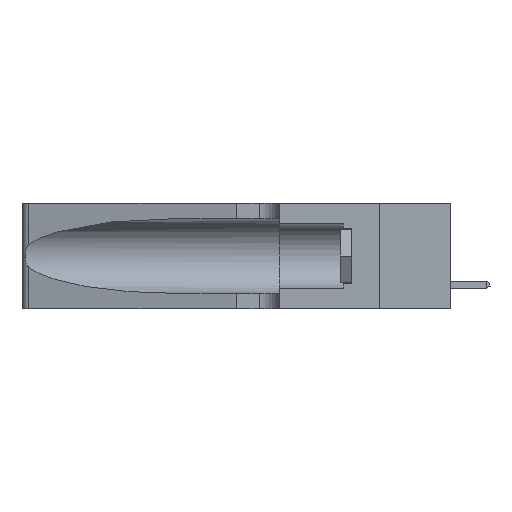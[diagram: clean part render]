
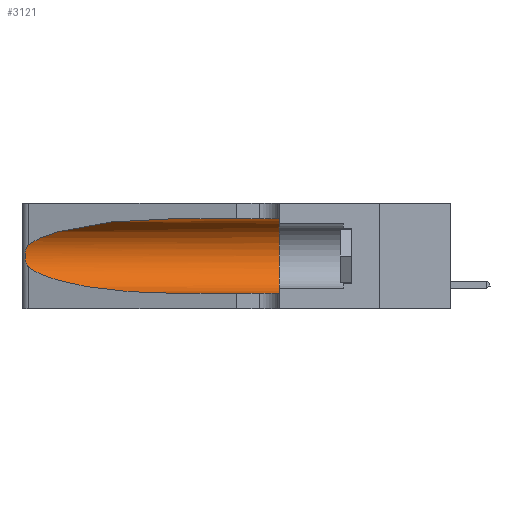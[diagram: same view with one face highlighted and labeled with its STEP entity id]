
A CAD part, left-side view. The second image highlights one B-rep face of the part: STEP entity #3121.
In plain terms, the highlighted cylindrical face has radius 3.308 mm (diameter 6.617 mm), a partial arc.
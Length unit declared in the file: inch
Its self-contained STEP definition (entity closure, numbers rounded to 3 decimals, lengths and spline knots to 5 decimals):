
#1227 = DIRECTION ( 'NONE',  ( 0., 1., 0. ) ) ;
#1298 = CYLINDRICAL_SURFACE ( 'NONE', #15451, 0.13025 ) ;
#1699 = CARTESIAN_POINT ( 'NONE',  ( 0.1305, 0.35, 0.05475 ) ) ;
#2047 = VERTEX_POINT ( 'NONE', #17541 ) ;
#2241 = ORIENTED_EDGE ( 'NONE', *, *, #7390, .F. ) ;
#3095 = CARTESIAN_POINT ( 'NONE',  ( 0.25487, 1.22718, 0.14631 ) ) ;
#3121 = ADVANCED_FACE ( 'NONE', ( #20986 ), #1298, .F. ) ;
#3146 = CARTESIAN_POINT ( 'NONE',  ( 0.18966, 0.96281, 0.05475 ) ) ;
#3394 = CARTESIAN_POINT ( 'NONE',  ( 0.25487, 1.22718, 0.22369 ) ) ;
#3983 = LINE ( 'NONE', #20571, #10694 ) ;
#4191 = CARTESIAN_POINT ( 'NONE',  ( 0.1305, 0.35, 0.31525 ) ) ;
#4752 = ORIENTED_EDGE ( 'NONE', *, *, #6547, .T. ) ;
#4838 = CARTESIAN_POINT ( 'NONE',  ( 0.26017, 1.23833, 0.17102 ) ) ;
#4986 = CARTESIAN_POINT ( 'NONE',  ( 0.25639, 1.23186, 0.15144 ) ) ;
#5048 = LINE ( 'NONE', #17758, #10994 ) ;
#5130 = CARTESIAN_POINT ( 'NONE',  ( 0.1305, 0.72297, 0.31525 ) ) ;
#5148 = VERTEX_POINT ( 'NONE', #4191 ) ;
#5257 = DIRECTION ( 'NONE',  ( 0., 0., 1. ) ) ;
#5874 = ORIENTED_EDGE ( 'NONE', *, *, #18581, .T. ) ;
#6061 = AXIS2_PLACEMENT_3D ( 'NONE', #8800, #1227, #5257 ) ;
#6135 = CARTESIAN_POINT ( 'NONE',  ( 0.25487, 1.22718, 0.14631 ) ) ;
#6547 = EDGE_CURVE ( 'NONE', #17490, #2047, #18963, .T. ) ;
#6557 = CARTESIAN_POINT ( 'NONE',  ( 0.25487, 1.22718, 0.14631 ) ) ;
#7006 = DIRECTION ( 'NONE',  ( 0., -1., 0. ) ) ;
#7390 = EDGE_CURVE ( 'NONE', #14608, #5148, #3983, .T. ) ;
#7505 = ORIENTED_EDGE ( 'NONE', *, *, #15614, .T. ) ;
#8241 = CARTESIAN_POINT ( 'NONE',  ( 0.26075, 1.23896, 0.178 ) ) ;
#8556 = B_SPLINE_CURVE_WITH_KNOTS ( 'NONE', 3,
 ( #3394, #14654, #14946, #11481, #13056, #16497, #18181, #8241, #4838, #9876, #21451, #4986, #16568, #3095 ),
 .UNSPECIFIED., .F., .F.,
 ( 4, 2, 2, 2, 2, 2, 4 ),
 ( 0., 0.00027, 0.00053, 0.00107, 0.0016, 0.00187, 0.00214 ),
 .UNSPECIFIED. ) ;
#8800 = CARTESIAN_POINT ( 'NONE',  ( 0.1305, 0.35, 0.185 ) ) ;
#9723 = CARTESIAN_POINT ( 'NONE',  ( 0.2373, 1.15595, 0.08982 ) ) ;
#9876 = CARTESIAN_POINT ( 'NONE',  ( 0.25856, 1.23593, 0.16098 ) ) ;
#10129 =( BOUNDED_CURVE ( )  B_SPLINE_CURVE ( 3, ( #11267, #16569, #16729, #15233 ),
 .UNSPECIFIED., .F., .F. ) 
 B_SPLINE_CURVE_WITH_KNOTS ( ( 4, 4 ),
 ( 1.5708, 2.84003 ),
 .UNSPECIFIED. ) 
 CURVE ( )  GEOMETRIC_REPRESENTATION_ITEM ( )  RATIONAL_B_SPLINE_CURVE ( ( 1., 0.87, 0.87, 1. ) ) 
 REPRESENTATION_ITEM ( '' )  );
#10694 = VECTOR ( 'NONE', #7006, 39.37008 ) ;
#10919 = DIRECTION ( 'NONE',  ( 0., -1., 0. ) ) ;
#10994 = VECTOR ( 'NONE', #19414, 39.37008 ) ;
#11267 = CARTESIAN_POINT ( 'NONE',  ( 0.1305, 0.72297, 0.31525 ) ) ;
#11481 = CARTESIAN_POINT ( 'NONE',  ( 0.25787, 1.23484, 0.2124 ) ) ;
#13056 = CARTESIAN_POINT ( 'NONE',  ( 0.25854, 1.2359, 0.20912 ) ) ;
#13141 = CIRCLE ( 'NONE', #6061, 0.13025 ) ;
#14025 = EDGE_LOOP ( 'NONE', ( #7505, #19685, #4752, #5874, #17867, #2241 ) ) ;
#14439 = CARTESIAN_POINT ( 'NONE',  ( 0.25487, 1.22718, 0.22369 ) ) ;
#14608 = VERTEX_POINT ( 'NONE', #5130 ) ;
#14654 = CARTESIAN_POINT ( 'NONE',  ( 0.25555, 1.22994, 0.2215 ) ) ;
#14946 = CARTESIAN_POINT ( 'NONE',  ( 0.25639, 1.23184, 0.21858 ) ) ;
#15233 = CARTESIAN_POINT ( 'NONE',  ( 0.25487, 1.22718, 0.22369 ) ) ;
#15451 = AXIS2_PLACEMENT_3D ( 'NONE', #15852, #10919, #20992 ) ;
#15614 = EDGE_CURVE ( 'NONE', #14608, #17600, #10129, .T. ) ;
#15852 = CARTESIAN_POINT ( 'NONE',  ( 0.1305, 1.61858, 0.185 ) ) ;
#15877 = EDGE_CURVE ( 'NONE', #5148, #19279, #13141, .T. ) ;
#16497 = CARTESIAN_POINT ( 'NONE',  ( 0.26018, 1.23835, 0.19895 ) ) ;
#16552 = CARTESIAN_POINT ( 'NONE',  ( 0.1305, 0.72297, 0.05475 ) ) ;
#16568 = CARTESIAN_POINT ( 'NONE',  ( 0.25555, 1.22993, 0.14849 ) ) ;
#16569 = CARTESIAN_POINT ( 'NONE',  ( 0.18966, 0.96281, 0.31525 ) ) ;
#16729 = CARTESIAN_POINT ( 'NONE',  ( 0.2373, 1.15595, 0.28018 ) ) ;
#17315 = EDGE_CURVE ( 'NONE', #17600, #17490, #8556, .T. ) ;
#17490 = VERTEX_POINT ( 'NONE', #6135 ) ;
#17541 = CARTESIAN_POINT ( 'NONE',  ( 0.1305, 0.72297, 0.05475 ) ) ;
#17600 = VERTEX_POINT ( 'NONE', #14439 ) ;
#17758 = CARTESIAN_POINT ( 'NONE',  ( 0.1305, 1.61858, 0.05475 ) ) ;
#17867 = ORIENTED_EDGE ( 'NONE', *, *, #15877, .F. ) ;
#18181 = CARTESIAN_POINT ( 'NONE',  ( 0.26075, 1.23896, 0.19203 ) ) ;
#18581 = EDGE_CURVE ( 'NONE', #2047, #19279, #5048, .T. ) ;
#18963 =( BOUNDED_CURVE ( )  B_SPLINE_CURVE ( 3, ( #6557, #9723, #3146, #16552 ),
 .UNSPECIFIED., .F., .T. ) 
 B_SPLINE_CURVE_WITH_KNOTS ( ( 4, 4 ),
 ( 3.44316, 4.71239 ),
 .UNSPECIFIED. ) 
 CURVE ( )  GEOMETRIC_REPRESENTATION_ITEM ( )  RATIONAL_B_SPLINE_CURVE ( ( 1., 0.87, 0.87, 1. ) ) 
 REPRESENTATION_ITEM ( '' )  );
#19279 = VERTEX_POINT ( 'NONE', #1699 ) ;
#19414 = DIRECTION ( 'NONE',  ( 0., -1., 0. ) ) ;
#19685 = ORIENTED_EDGE ( 'NONE', *, *, #17315, .T. ) ;
#20571 = CARTESIAN_POINT ( 'NONE',  ( 0.1305, 1.61858, 0.31525 ) ) ;
#20986 = FACE_OUTER_BOUND ( 'NONE', #14025, .T. ) ;
#20992 = DIRECTION ( 'NONE',  ( 0., 0., -1. ) ) ;
#21451 = CARTESIAN_POINT ( 'NONE',  ( 0.25789, 1.23486, 0.15765 ) ) ;
